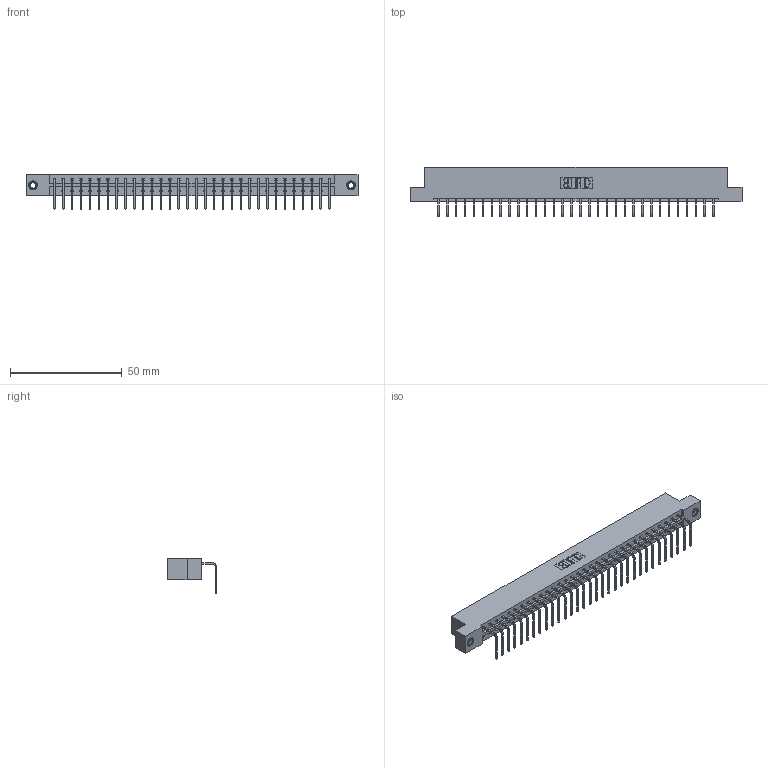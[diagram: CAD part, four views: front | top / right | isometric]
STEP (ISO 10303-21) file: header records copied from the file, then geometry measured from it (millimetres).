
FILE_DESCRIPTION (( 'STEP AP203' ), '1' );
FILE_NAME ('333-032-558-107.STEP', '2018-08-02T20:39:05', ( '' ), ( '' ), 'SwSTEP 2.0', 'SolidWorks 2016', '' );
FILE_SCHEMA (( 'CONFIG_CONTROL_DESIGN' ));
Length unit declared in the file: inch
Products named in the file (4): 345-292-001_558 Tail - 2; 345-250-001_345-250-005-103; 333-032-558-107; 333 Part_Flush - .156 Dia - TI
Assembly tree (35 placements, depth 2):
  333-032-558-107
    333 Part_Flush - .156 Dia - TI
    345-292-001_558 Tail - 2  x32
    345-250-001_345-250-005-103  x2
Bounding box: 148.34 x 22.17 x 15.37 mm (x, y, z)
Volume: 14933.9 mm3; surface area: 16784.1 mm2
Topology: 35 solids, 35 shells, 2094 faces, 6271 edges, 4130 vertices
Faces by surface type: plane 1510, cylinder 568, cone 12, torus 4
Entity records: 22126 total; most frequent: CARTESIAN_POINT 3801, ORIENTED_EDGE 3762, DIRECTION 3259, EDGE_CURVE 1881, LINE 1733, VECTOR 1733, VERTEX_POINT 1248, AXIS2_PLACEMENT_3D 763
